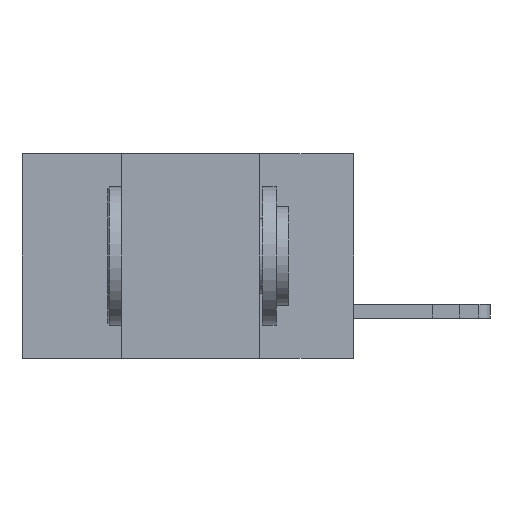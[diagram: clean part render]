
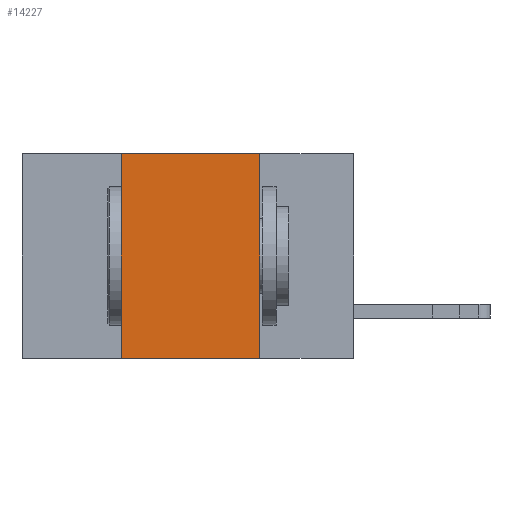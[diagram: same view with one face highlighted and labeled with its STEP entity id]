
A CAD part, left-side view. The second image highlights one B-rep face of the part: STEP entity #14227.
In plain terms, the highlighted planar face has unit normal (-1, 0, 0).
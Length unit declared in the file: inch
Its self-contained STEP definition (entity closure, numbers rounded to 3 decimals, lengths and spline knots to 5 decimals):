
#532 = LINE ( 'NONE', #9408, #11982 ) ;
#1533 = VECTOR ( 'NONE', #15103, 39.37008 ) ;
#1785 = ORIENTED_EDGE ( 'NONE', *, *, #14332, .F. ) ;
#1844 = VERTEX_POINT ( 'NONE', #5297 ) ;
#2350 = ORIENTED_EDGE ( 'NONE', *, *, #14802, .F. ) ;
#3182 = LINE ( 'NONE', #8590, #1533 ) ;
#3698 = ORIENTED_EDGE ( 'NONE', *, *, #8435, .F. ) ;
#4663 = VERTEX_POINT ( 'NONE', #7616 ) ;
#5297 = CARTESIAN_POINT ( 'NONE',  ( 0., 0.42, 0. ) ) ;
#5519 = VECTOR ( 'NONE', #10885, 39.37008 ) ;
#5978 = FACE_OUTER_BOUND ( 'NONE', #12550, .T. ) ;
#6086 = VECTOR ( 'NONE', #11124, 39.37008 ) ;
#7401 = CARTESIAN_POINT ( 'NONE',  ( 0., 0.6, 0. ) ) ;
#7573 = PLANE ( 'NONE',  #9665 ) ;
#7616 = CARTESIAN_POINT ( 'NONE',  ( 0., 0.17, -0.37 ) ) ;
#7661 = DIRECTION ( 'NONE',  ( 1., 0., 0. ) ) ;
#7899 = CARTESIAN_POINT ( 'NONE',  ( 0., 0.17, 0. ) ) ;
#8156 = LINE ( 'NONE', #12206, #5519 ) ;
#8286 = CARTESIAN_POINT ( 'NONE',  ( 0., 0.42, -0.37 ) ) ;
#8318 = EDGE_CURVE ( 'NONE', #12363, #4663, #8156, .T. ) ;
#8435 = EDGE_CURVE ( 'NONE', #12363, #1844, #3182, .T. ) ;
#8590 = CARTESIAN_POINT ( 'NONE',  ( 0., 0.42, 0. ) ) ;
#9408 = CARTESIAN_POINT ( 'NONE',  ( 0., 0.6, 0. ) ) ;
#9665 = AXIS2_PLACEMENT_3D ( 'NONE', #7401, #7661, #11610 ) ;
#10885 = DIRECTION ( 'NONE',  ( 0., -1., 0. ) ) ;
#11043 = CARTESIAN_POINT ( 'NONE',  ( 0., 0.17, 0. ) ) ;
#11124 = DIRECTION ( 'NONE',  ( 0., 0., -1. ) ) ;
#11610 = DIRECTION ( 'NONE',  ( 0., 0., -1. ) ) ;
#11982 = VECTOR ( 'NONE', #14714, 39.37008 ) ;
#12206 = CARTESIAN_POINT ( 'NONE',  ( 0., 0.6, -0.37 ) ) ;
#12363 = VERTEX_POINT ( 'NONE', #8286 ) ;
#12550 = EDGE_LOOP ( 'NONE', ( #2350, #1785, #3698, #12996 ) ) ;
#12996 = ORIENTED_EDGE ( 'NONE', *, *, #8318, .T. ) ;
#13544 = VERTEX_POINT ( 'NONE', #7899 ) ;
#14227 = ADVANCED_FACE ( 'NONE', ( #5978 ), #7573, .F. ) ;
#14332 = EDGE_CURVE ( 'NONE', #1844, #13544, #532, .T. ) ;
#14714 = DIRECTION ( 'NONE',  ( 0., -1., 0. ) ) ;
#14802 = EDGE_CURVE ( 'NONE', #13544, #4663, #15090, .T. ) ;
#15090 = LINE ( 'NONE', #11043, #6086 ) ;
#15103 = DIRECTION ( 'NONE',  ( 0., 0., 1. ) ) ;
